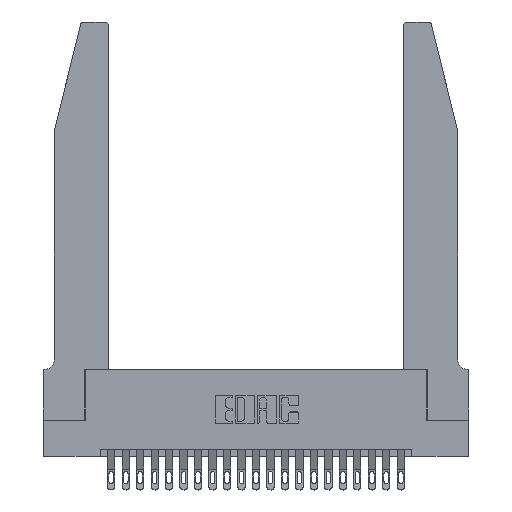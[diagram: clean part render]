
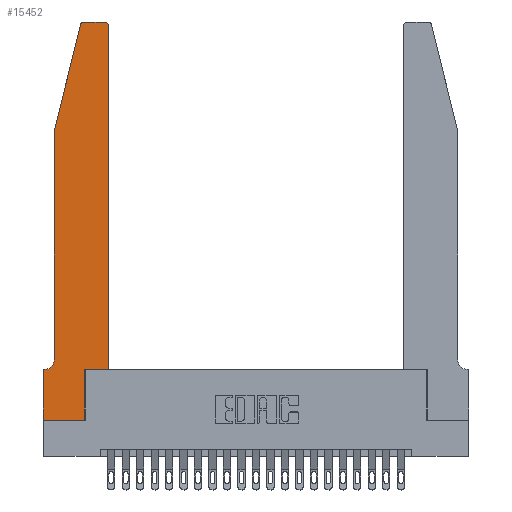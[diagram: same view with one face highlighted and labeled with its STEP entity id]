
A CAD part, top view. The second image highlights one B-rep face of the part: STEP entity #15452.
In plain terms, the highlighted planar face has unit normal (0, 0, 1).
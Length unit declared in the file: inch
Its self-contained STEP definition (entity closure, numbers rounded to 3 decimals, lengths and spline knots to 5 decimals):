
#201 = DIRECTION ( 'NONE',  ( 0., 0., 1. ) ) ;
#385 = DIRECTION ( 'NONE',  ( 0., 0., 1. ) ) ;
#477 = CARTESIAN_POINT ( 'NONE',  ( 0.2865, 0.35, 0.37 ) ) ;
#802 = CARTESIAN_POINT ( 'NONE',  ( 0.284, 2.75, 0.37 ) ) ;
#833 = AXIS2_PLACEMENT_3D ( 'NONE', #8911, #21936, #10811 ) ;
#1135 = DIRECTION ( 'NONE',  ( -0.239, -0.971, 0. ) ) ;
#1172 = VERTEX_POINT ( 'NONE', #802 ) ;
#1286 = VECTOR ( 'NONE', #15687, 39.37008 ) ;
#1336 = EDGE_CURVE ( 'NONE', #23224, #15636, #20933, .T. ) ;
#1483 = LINE ( 'NONE', #12431, #17197 ) ;
#1764 = LINE ( 'NONE', #11790, #11378 ) ;
#1967 = CARTESIAN_POINT ( 'NONE',  ( 0.4505, 0.35, 0.37 ) ) ;
#2438 = CIRCLE ( 'NONE', #5776, 0.03 ) ;
#2720 = DIRECTION ( 'NONE',  ( 0., -1., 0. ) ) ;
#2981 = ORIENTED_EDGE ( 'NONE', *, *, #9076, .T. ) ;
#3100 = ORIENTED_EDGE ( 'NONE', *, *, #11155, .T. ) ;
#3596 = EDGE_CURVE ( 'NONE', #20448, #5351, #4166, .T. ) ;
#4036 = CARTESIAN_POINT ( 'NONE',  ( 0.4505, 2.72, 0.37 ) ) ;
#4166 = LINE ( 'NONE', #19976, #23513 ) ;
#4556 = DIRECTION ( 'NONE',  ( 1., 0., 0. ) ) ;
#4657 = LINE ( 'NONE', #18816, #23977 ) ;
#5351 = VERTEX_POINT ( 'NONE', #19355 ) ;
#5574 = EDGE_LOOP ( 'NONE', ( #3100, #18412, #11909, #11598, #18211, #17538, #9501, #20351, #9006, #2981, #12539, #19337 ) ) ;
#5672 = CARTESIAN_POINT ( 'NONE',  ( 0., 0.35, 0.37 ) ) ;
#5776 = AXIS2_PLACEMENT_3D ( 'NONE', #11860, #385, #13738 ) ;
#5891 = VERTEX_POINT ( 'NONE', #1967 ) ;
#7175 = LINE ( 'NONE', #10764, #12174 ) ;
#7182 = EDGE_CURVE ( 'NONE', #15636, #20759, #12677, .T. ) ;
#7239 = CIRCLE ( 'NONE', #833, 0.07 ) ;
#7607 = DIRECTION ( 'NONE',  ( 1., 0., 0. ) ) ;
#7825 = VECTOR ( 'NONE', #4556, 39.37008 ) ;
#8911 = CARTESIAN_POINT ( 'NONE',  ( 0.0055, 0.42, 0.37 ) ) ;
#9006 = ORIENTED_EDGE ( 'NONE', *, *, #7182, .T. ) ;
#9076 = EDGE_CURVE ( 'NONE', #20759, #5891, #13434, .T. ) ;
#9424 = PLANE ( 'NONE',  #20057 ) ;
#9501 = ORIENTED_EDGE ( 'NONE', *, *, #22663, .T. ) ;
#10242 = VERTEX_POINT ( 'NONE', #19772 ) ;
#10587 = DIRECTION ( 'NONE',  ( -1., 0., 0. ) ) ;
#10608 = EDGE_CURVE ( 'NONE', #5351, #10242, #1764, .T. ) ;
#10651 = DIRECTION ( 'NONE',  ( 1., 0., 0. ) ) ;
#10709 = CARTESIAN_POINT ( 'NONE',  ( 0., 0., 0.37 ) ) ;
#10764 = CARTESIAN_POINT ( 'NONE',  ( 0.4505, 0.35, 0.37 ) ) ;
#10811 = DIRECTION ( 'NONE',  ( -1., 0., 0. ) ) ;
#10845 = EDGE_CURVE ( 'NONE', #10242, #22337, #7239, .T. ) ;
#11108 = LINE ( 'NONE', #21696, #15442 ) ;
#11155 = EDGE_CURVE ( 'NONE', #12892, #1172, #11108, .T. ) ;
#11178 = FACE_OUTER_BOUND ( 'NONE', #5574, .T. ) ;
#11378 = VECTOR ( 'NONE', #15514, 39.37008 ) ;
#11565 = VERTEX_POINT ( 'NONE', #4036 ) ;
#11598 = ORIENTED_EDGE ( 'NONE', *, *, #10608, .T. ) ;
#11687 = CARTESIAN_POINT ( 'NONE',  ( 0.4205, 2.72, 0.37 ) ) ;
#11790 = CARTESIAN_POINT ( 'NONE',  ( 0.0755, 2., 0.37 ) ) ;
#11860 = CARTESIAN_POINT ( 'NONE',  ( 0.284, 2.72, 0.37 ) ) ;
#11909 = ORIENTED_EDGE ( 'NONE', *, *, #3596, .T. ) ;
#12174 = VECTOR ( 'NONE', #21881, 39.37008 ) ;
#12431 = CARTESIAN_POINT ( 'NONE',  ( 0., 0., 0.37 ) ) ;
#12539 = ORIENTED_EDGE ( 'NONE', *, *, #17600, .T. ) ;
#12677 = LINE ( 'NONE', #477, #1286 ) ;
#12858 = VECTOR ( 'NONE', #10651, 39.37008 ) ;
#12892 = VERTEX_POINT ( 'NONE', #17553 ) ;
#13434 = LINE ( 'NONE', #23622, #12858 ) ;
#13565 = DIRECTION ( 'NONE',  ( 1., 0., 0. ) ) ;
#13738 = DIRECTION ( 'NONE',  ( 1., 0., 0. ) ) ;
#14467 = CIRCLE ( 'NONE', #22110, 0.03 ) ;
#14832 = EDGE_CURVE ( 'NONE', #22337, #17901, #4657, .T. ) ;
#15442 = VECTOR ( 'NONE', #10587, 39.37008 ) ;
#15452 = ADVANCED_FACE ( 'NONE', ( #11178 ), #9424, .T. ) ;
#15514 = DIRECTION ( 'NONE',  ( 0., -1., 0. ) ) ;
#15622 = EDGE_CURVE ( 'NONE', #1172, #20448, #2438, .T. ) ;
#15636 = VERTEX_POINT ( 'NONE', #22982 ) ;
#15687 = DIRECTION ( 'NONE',  ( 0., 1., 0. ) ) ;
#17197 = VECTOR ( 'NONE', #2720, 39.37008 ) ;
#17538 = ORIENTED_EDGE ( 'NONE', *, *, #14832, .T. ) ;
#17553 = CARTESIAN_POINT ( 'NONE',  ( 0.4205, 2.75, 0.37 ) ) ;
#17600 = EDGE_CURVE ( 'NONE', #5891, #11565, #7175, .T. ) ;
#17901 = VERTEX_POINT ( 'NONE', #20880 ) ;
#18211 = ORIENTED_EDGE ( 'NONE', *, *, #10845, .T. ) ;
#18412 = ORIENTED_EDGE ( 'NONE', *, *, #15622, .T. ) ;
#18502 = EDGE_CURVE ( 'NONE', #11565, #12892, #14467, .T. ) ;
#18790 = DIRECTION ( 'NONE',  ( 0., 0., 1. ) ) ;
#18816 = CARTESIAN_POINT ( 'NONE',  ( 0.0755, 0.35, 0.37 ) ) ;
#18895 = DIRECTION ( 'NONE',  ( -1., 0., 0. ) ) ;
#19337 = ORIENTED_EDGE ( 'NONE', *, *, #18502, .T. ) ;
#19355 = CARTESIAN_POINT ( 'NONE',  ( 0.0755, 2., 0.37 ) ) ;
#19772 = CARTESIAN_POINT ( 'NONE',  ( 0.0755, 0.42, 0.37 ) ) ;
#19976 = CARTESIAN_POINT ( 'NONE',  ( 0.0755, 2., 0.37 ) ) ;
#20057 = AXIS2_PLACEMENT_3D ( 'NONE', #5672, #18790, #7607 ) ;
#20351 = ORIENTED_EDGE ( 'NONE', *, *, #1336, .T. ) ;
#20448 = VERTEX_POINT ( 'NONE', #21346 ) ;
#20596 = CARTESIAN_POINT ( 'NONE',  ( 0.2865, 0.35, 0.37 ) ) ;
#20759 = VERTEX_POINT ( 'NONE', #20596 ) ;
#20880 = CARTESIAN_POINT ( 'NONE',  ( 0., 0.35, 0.37 ) ) ;
#20933 = LINE ( 'NONE', #10709, #7825 ) ;
#21346 = CARTESIAN_POINT ( 'NONE',  ( 0.25487, 2.72718, 0.37 ) ) ;
#21413 = CARTESIAN_POINT ( 'NONE',  ( 0., 0., 0.37 ) ) ;
#21696 = CARTESIAN_POINT ( 'NONE',  ( 0.2605, 2.75, 0.37 ) ) ;
#21881 = DIRECTION ( 'NONE',  ( 0., 1., 0. ) ) ;
#21936 = DIRECTION ( 'NONE',  ( 0., 0., -1. ) ) ;
#22110 = AXIS2_PLACEMENT_3D ( 'NONE', #11687, #201, #13565 ) ;
#22337 = VERTEX_POINT ( 'NONE', #22658 ) ;
#22658 = CARTESIAN_POINT ( 'NONE',  ( 0.0055, 0.35, 0.37 ) ) ;
#22663 = EDGE_CURVE ( 'NONE', #17901, #23224, #1483, .T. ) ;
#22982 = CARTESIAN_POINT ( 'NONE',  ( 0.2865, 0., 0.37 ) ) ;
#23224 = VERTEX_POINT ( 'NONE', #21413 ) ;
#23513 = VECTOR ( 'NONE', #1135, 39.37008 ) ;
#23622 = CARTESIAN_POINT ( 'NONE',  ( 0.4505, 0.35, 0.37 ) ) ;
#23977 = VECTOR ( 'NONE', #18895, 39.37008 ) ;
